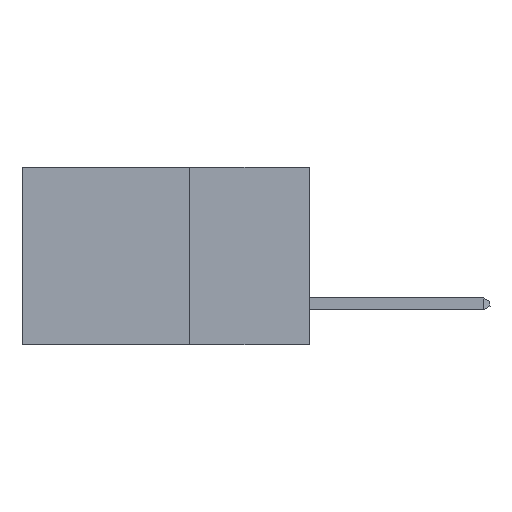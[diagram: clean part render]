
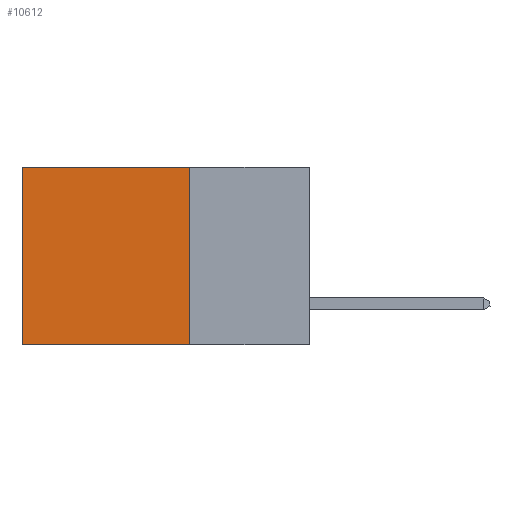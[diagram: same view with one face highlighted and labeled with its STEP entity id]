
A CAD part, left-side view. The second image highlights one B-rep face of the part: STEP entity #10612.
In plain terms, the highlighted planar face has unit normal (-1, 0, 0).
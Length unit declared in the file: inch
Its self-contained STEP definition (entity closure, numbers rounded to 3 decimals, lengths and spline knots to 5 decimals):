
#302 = CARTESIAN_POINT ( 'NONE',  ( 0.2875, 0.25, 0. ) ) ;
#326 = CARTESIAN_POINT ( 'NONE',  ( 0.2875, 0.25, 0. ) ) ;
#961 = VECTOR ( 'NONE', #2672, 39.37008 ) ;
#1336 = ORIENTED_EDGE ( 'NONE', *, *, #8485, .F. ) ;
#2672 = DIRECTION ( 'NONE',  ( 0., 0., -1. ) ) ;
#3161 = CARTESIAN_POINT ( 'NONE',  ( 0.2875, 0.25, -0.37 ) ) ;
#3516 = ORIENTED_EDGE ( 'NONE', *, *, #8035, .T. ) ;
#3523 = LINE ( 'NONE', #3161, #22198 ) ;
#4752 = ORIENTED_EDGE ( 'NONE', *, *, #25366, .T. ) ;
#4889 = LINE ( 'NONE', #20654, #16601 ) ;
#4906 = CARTESIAN_POINT ( 'NONE',  ( 0.2875, 0.25, -0.37 ) ) ;
#4913 = DIRECTION ( 'NONE',  ( 0., 0., -1. ) ) ;
#6901 = CARTESIAN_POINT ( 'NONE',  ( 0.2875, 0.6, 0. ) ) ;
#8035 = EDGE_CURVE ( 'NONE', #8566, #27393, #18826, .T. ) ;
#8189 = VECTOR ( 'NONE', #18948, 39.37008 ) ;
#8485 = EDGE_CURVE ( 'NONE', #12556, #17650, #4889, .T. ) ;
#8528 = FACE_OUTER_BOUND ( 'NONE', #13832, .T. ) ;
#8566 = VERTEX_POINT ( 'NONE', #6901 ) ;
#10612 = ADVANCED_FACE ( 'NONE', ( #8528 ), #28358, .F. ) ;
#12556 = VERTEX_POINT ( 'NONE', #14664 ) ;
#13347 = ORIENTED_EDGE ( 'NONE', *, *, #19350, .F. ) ;
#13692 = DIRECTION ( 'NONE',  ( 0., 0., -1. ) ) ;
#13832 = EDGE_LOOP ( 'NONE', ( #3516, #13347, #1336, #4752 ) ) ;
#14664 = CARTESIAN_POINT ( 'NONE',  ( 0.2875, 0.25, 0. ) ) ;
#16601 = VECTOR ( 'NONE', #13692, 39.37008 ) ;
#17650 = VERTEX_POINT ( 'NONE', #4906 ) ;
#18315 = AXIS2_PLACEMENT_3D ( 'NONE', #302, #18929, #4913 ) ;
#18826 = LINE ( 'NONE', #19009, #961 ) ;
#18929 = DIRECTION ( 'NONE',  ( 1., 0., 0. ) ) ;
#18948 = DIRECTION ( 'NONE',  ( 0., 1., 0. ) ) ;
#19009 = CARTESIAN_POINT ( 'NONE',  ( 0.2875, 0.6, 0. ) ) ;
#19350 = EDGE_CURVE ( 'NONE', #17650, #27393, #3523, .T. ) ;
#19507 = DIRECTION ( 'NONE',  ( 0., 1., 0. ) ) ;
#19923 = CARTESIAN_POINT ( 'NONE',  ( 0.2875, 0.6, -0.37 ) ) ;
#20654 = CARTESIAN_POINT ( 'NONE',  ( 0.2875, 0.25, 0. ) ) ;
#20680 = LINE ( 'NONE', #326, #8189 ) ;
#22198 = VECTOR ( 'NONE', #19507, 39.37008 ) ;
#25366 = EDGE_CURVE ( 'NONE', #12556, #8566, #20680, .T. ) ;
#27393 = VERTEX_POINT ( 'NONE', #19923 ) ;
#28358 = PLANE ( 'NONE',  #18315 ) ;
